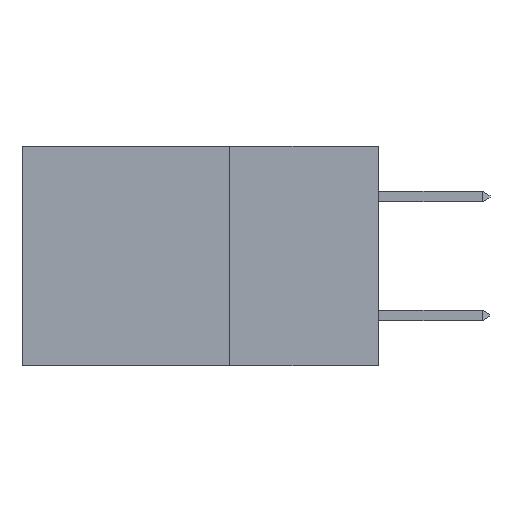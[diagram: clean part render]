
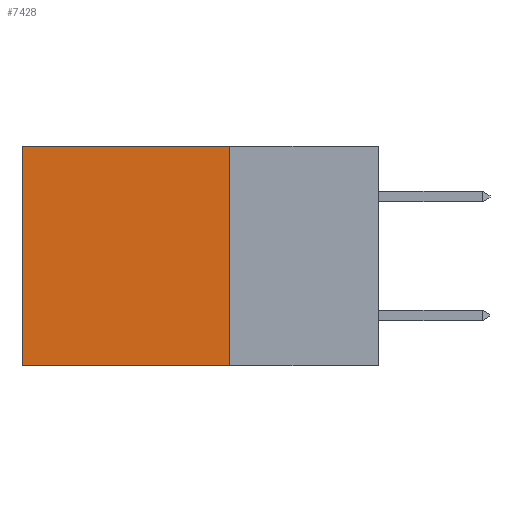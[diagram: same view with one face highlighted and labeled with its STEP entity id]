
A CAD part, left-side view. The second image highlights one B-rep face of the part: STEP entity #7428.
In plain terms, the highlighted planar face has unit normal (-1, 0, 0).
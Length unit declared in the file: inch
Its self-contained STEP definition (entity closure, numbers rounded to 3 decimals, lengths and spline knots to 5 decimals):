
#55 = VECTOR ( 'NONE', #6391, 39.37008 ) ;
#500 = CARTESIAN_POINT ( 'NONE',  ( 0.298, 0.25, 0. ) ) ;
#1658 = VECTOR ( 'NONE', #6093, 39.37008 ) ;
#1847 = VECTOR ( 'NONE', #2894, 39.37008 ) ;
#1969 = CARTESIAN_POINT ( 'NONE',  ( 0.298, 0.25, -0.37 ) ) ;
#2894 = DIRECTION ( 'NONE',  ( 0., 0., -1. ) ) ;
#2909 = VERTEX_POINT ( 'NONE', #6471 ) ;
#2957 = EDGE_CURVE ( 'NONE', #10888, #7767, #11327, .T. ) ;
#2968 = DIRECTION ( 'NONE',  ( 1., 0., 0. ) ) ;
#3048 = EDGE_CURVE ( 'NONE', #2909, #5911, #5287, .T. ) ;
#3349 = ORIENTED_EDGE ( 'NONE', *, *, #3048, .T. ) ;
#3359 = ORIENTED_EDGE ( 'NONE', *, *, #2957, .F. ) ;
#4201 = FACE_OUTER_BOUND ( 'NONE', #6858, .T. ) ;
#4320 = LINE ( 'NONE', #9397, #1847 ) ;
#5287 = LINE ( 'NONE', #6338, #55 ) ;
#5543 = ORIENTED_EDGE ( 'NONE', *, *, #10515, .F. ) ;
#5911 = VERTEX_POINT ( 'NONE', #11679 ) ;
#6093 = DIRECTION ( 'NONE',  ( 0., 0., -1. ) ) ;
#6338 = CARTESIAN_POINT ( 'NONE',  ( 0.298, 0.25, 0. ) ) ;
#6391 = DIRECTION ( 'NONE',  ( 0., 1., 0. ) ) ;
#6471 = CARTESIAN_POINT ( 'NONE',  ( 0.298, 0.25, 0. ) ) ;
#6686 = PLANE ( 'NONE',  #9957 ) ;
#6858 = EDGE_LOOP ( 'NONE', ( #10394, #3359, #5543, #3349 ) ) ;
#7428 = ADVANCED_FACE ( 'NONE', ( #4201 ), #6686, .F. ) ;
#7767 = VERTEX_POINT ( 'NONE', #11827 ) ;
#8242 = DIRECTION ( 'NONE',  ( 0., 1., 0. ) ) ;
#8401 = VECTOR ( 'NONE', #8242, 39.37008 ) ;
#8552 = CARTESIAN_POINT ( 'NONE',  ( 0.298, 0.25, 0. ) ) ;
#8580 = EDGE_CURVE ( 'NONE', #5911, #7767, #4320, .T. ) ;
#9397 = CARTESIAN_POINT ( 'NONE',  ( 0.298, 0.6, 0. ) ) ;
#9459 = DIRECTION ( 'NONE',  ( 0., 0., -1. ) ) ;
#9957 = AXIS2_PLACEMENT_3D ( 'NONE', #8552, #2968, #9459 ) ;
#10394 = ORIENTED_EDGE ( 'NONE', *, *, #8580, .T. ) ;
#10515 = EDGE_CURVE ( 'NONE', #2909, #10888, #11421, .T. ) ;
#10888 = VERTEX_POINT ( 'NONE', #1969 ) ;
#10906 = CARTESIAN_POINT ( 'NONE',  ( 0.298, 0.25, -0.37 ) ) ;
#11327 = LINE ( 'NONE', #10906, #8401 ) ;
#11421 = LINE ( 'NONE', #500, #1658 ) ;
#11679 = CARTESIAN_POINT ( 'NONE',  ( 0.298, 0.6, 0. ) ) ;
#11827 = CARTESIAN_POINT ( 'NONE',  ( 0.298, 0.6, -0.37 ) ) ;
